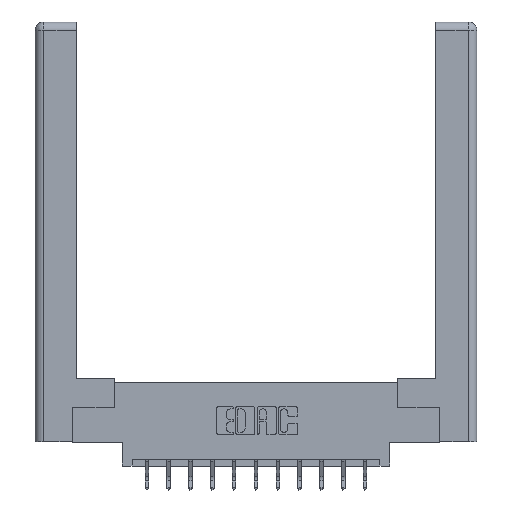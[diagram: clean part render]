
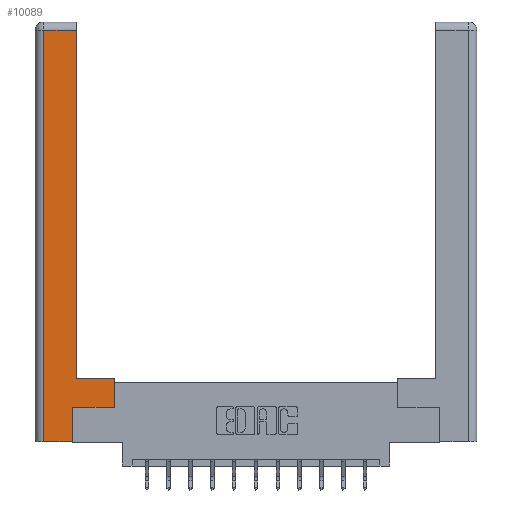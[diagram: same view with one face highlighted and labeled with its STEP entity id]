
A CAD part, top view. The second image highlights one B-rep face of the part: STEP entity #10089.
In plain terms, the highlighted planar face has unit normal (0, 0, 1).
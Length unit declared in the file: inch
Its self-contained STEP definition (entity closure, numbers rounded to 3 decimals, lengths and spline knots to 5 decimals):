
#1161 = CARTESIAN_POINT ( 'NONE',  ( 0.0615, 2.94, 0. ) ) ;
#1450 = EDGE_CURVE ( 'NONE', #10084, #9556, #3553, .T. ) ;
#1457 = ORIENTED_EDGE ( 'NONE', *, *, #7098, .T. ) ;
#1556 = LINE ( 'NONE', #10826, #4194 ) ;
#1688 = DIRECTION ( 'NONE',  ( 1., 0., 0. ) ) ;
#2117 = DIRECTION ( 'NONE',  ( 0., 0., -1. ) ) ;
#2176 = PLANE ( 'NONE',  #11286 ) ;
#2387 = EDGE_CURVE ( 'NONE', #11530, #2738, #5624, .T. ) ;
#2738 = VERTEX_POINT ( 'NONE', #8711 ) ;
#3206 = LINE ( 'NONE', #10740, #12426 ) ;
#3217 = ORIENTED_EDGE ( 'NONE', *, *, #1450, .T. ) ;
#3381 = CARTESIAN_POINT ( 'NONE',  ( 0.295, 2.94, 0. ) ) ;
#3432 = CARTESIAN_POINT ( 'NONE',  ( 0.265, 0.245, 0. ) ) ;
#3553 = LINE ( 'NONE', #14805, #14102 ) ;
#4194 = VECTOR ( 'NONE', #8415, 39.37008 ) ;
#4295 = EDGE_CURVE ( 'NONE', #6717, #11530, #7636, .T. ) ;
#4588 = CARTESIAN_POINT ( 'NONE',  ( 0.565, 0.45, 0. ) ) ;
#5624 = LINE ( 'NONE', #12964, #9392 ) ;
#6123 = EDGE_CURVE ( 'NONE', #2738, #14231, #1556, .T. ) ;
#6717 = VERTEX_POINT ( 'NONE', #3381 ) ;
#6939 = CARTESIAN_POINT ( 'NONE',  ( 0.565, 0.245, 0. ) ) ;
#7098 = EDGE_CURVE ( 'NONE', #14231, #10084, #3206, .T. ) ;
#7431 = EDGE_CURVE ( 'NONE', #10500, #6717, #11313, .T. ) ;
#7636 = LINE ( 'NONE', #10078, #8387 ) ;
#8118 = ORIENTED_EDGE ( 'NONE', *, *, #7431, .T. ) ;
#8306 = DIRECTION ( 'NONE',  ( 0., -1., 0. ) ) ;
#8387 = VECTOR ( 'NONE', #15023, 39.37008 ) ;
#8415 = DIRECTION ( 'NONE',  ( 1., 0., 0. ) ) ;
#8711 = CARTESIAN_POINT ( 'NONE',  ( 0.0615, 0., 0. ) ) ;
#9171 = CARTESIAN_POINT ( 'NONE',  ( 0.295, 0.45, 0. ) ) ;
#9392 = VECTOR ( 'NONE', #8306, 39.37008 ) ;
#9405 = DIRECTION ( 'NONE',  ( -1., 0., 0. ) ) ;
#9431 = EDGE_CURVE ( 'NONE', #9556, #9578, #13488, .T. ) ;
#9556 = VERTEX_POINT ( 'NONE', #6939 ) ;
#9578 = VERTEX_POINT ( 'NONE', #4588 ) ;
#9694 = DIRECTION ( 'NONE',  ( 0., 1., 0. ) ) ;
#10078 = CARTESIAN_POINT ( 'NONE',  ( 0.0615, 2.94, 0. ) ) ;
#10084 = VERTEX_POINT ( 'NONE', #3432 ) ;
#10089 = ADVANCED_FACE ( 'NONE', ( #13809 ), #2176, .F. ) ;
#10250 = ORIENTED_EDGE ( 'NONE', *, *, #11526, .T. ) ;
#10317 = VECTOR ( 'NONE', #12828, 39.37008 ) ;
#10500 = VERTEX_POINT ( 'NONE', #9171 ) ;
#10740 = CARTESIAN_POINT ( 'NONE',  ( 0.265, 0.245, 0. ) ) ;
#10826 = CARTESIAN_POINT ( 'NONE',  ( 0.265, 0., 0. ) ) ;
#10896 = CARTESIAN_POINT ( 'NONE',  ( 0.295, 0.45, 0. ) ) ;
#11111 = VECTOR ( 'NONE', #11541, 39.37008 ) ;
#11286 = AXIS2_PLACEMENT_3D ( 'NONE', #11745, #2117, #9405 ) ;
#11313 = LINE ( 'NONE', #13917, #11111 ) ;
#11394 = EDGE_LOOP ( 'NONE', ( #8118, #13674, #12434, #11449, #1457, #3217, #15191, #10250 ) ) ;
#11449 = ORIENTED_EDGE ( 'NONE', *, *, #6123, .T. ) ;
#11526 = EDGE_CURVE ( 'NONE', #9578, #10500, #14876, .T. ) ;
#11530 = VERTEX_POINT ( 'NONE', #1161 ) ;
#11541 = DIRECTION ( 'NONE',  ( 0., 1., 0. ) ) ;
#11583 = CARTESIAN_POINT ( 'NONE',  ( 0.565, 0.45, 0. ) ) ;
#11745 = CARTESIAN_POINT ( 'NONE',  ( 0., 0., 0. ) ) ;
#12426 = VECTOR ( 'NONE', #9694, 39.37008 ) ;
#12434 = ORIENTED_EDGE ( 'NONE', *, *, #2387, .T. ) ;
#12828 = DIRECTION ( 'NONE',  ( 0., 1., 0. ) ) ;
#12964 = CARTESIAN_POINT ( 'NONE',  ( 0.0615, 0., 0. ) ) ;
#13293 = DIRECTION ( 'NONE',  ( -1., 0., 0. ) ) ;
#13488 = LINE ( 'NONE', #11583, #10317 ) ;
#13674 = ORIENTED_EDGE ( 'NONE', *, *, #4295, .T. ) ;
#13809 = FACE_OUTER_BOUND ( 'NONE', #11394, .T. ) ;
#13917 = CARTESIAN_POINT ( 'NONE',  ( 0.295, 3., 0. ) ) ;
#14102 = VECTOR ( 'NONE', #1688, 39.37008 ) ;
#14231 = VERTEX_POINT ( 'NONE', #15207 ) ;
#14693 = VECTOR ( 'NONE', #13293, 39.37008 ) ;
#14805 = CARTESIAN_POINT ( 'NONE',  ( 0.565, 0.245, 0. ) ) ;
#14876 = LINE ( 'NONE', #10896, #14693 ) ;
#15023 = DIRECTION ( 'NONE',  ( -1., 0., 0. ) ) ;
#15191 = ORIENTED_EDGE ( 'NONE', *, *, #9431, .T. ) ;
#15207 = CARTESIAN_POINT ( 'NONE',  ( 0.265, 0., 0. ) ) ;
